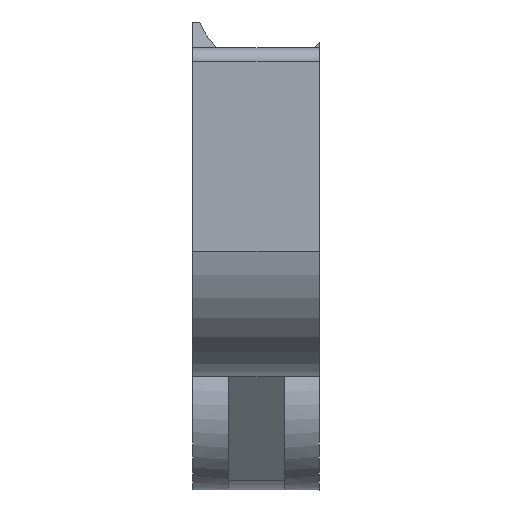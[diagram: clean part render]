
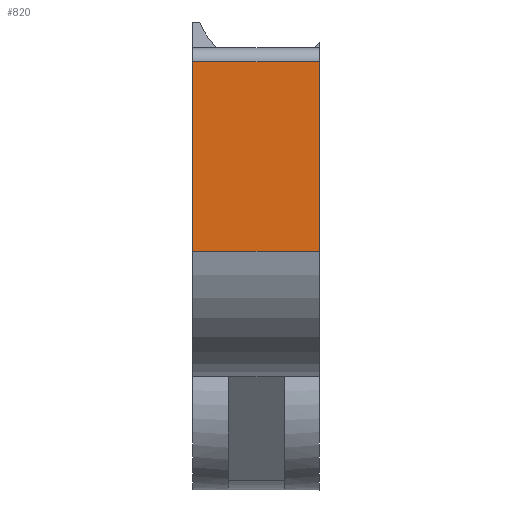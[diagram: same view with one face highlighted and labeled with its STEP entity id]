
A CAD part, left-side view. The second image highlights one B-rep face of the part: STEP entity #820.
In plain terms, the highlighted planar face has unit normal (-1, 0, 0).
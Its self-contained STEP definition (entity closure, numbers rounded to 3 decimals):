
#2 = DIRECTION ( 'NONE',  ( 0., -1., 0. ) ) ;
#34 = PLANE ( 'NONE',  #35 ) ;
#35 = AXIS2_PLACEMENT_3D ( 'NONE', #679, #856, #134 ) ;
#114 = EDGE_CURVE ( 'NONE', #207, #745, #587, .T. ) ;
#118 = DIRECTION ( 'NONE',  ( 0., 0., -1. ) ) ;
#122 = VECTOR ( 'NONE', #557, 1000. ) ;
#124 = ORIENTED_EDGE ( 'NONE', *, *, #149, .T. ) ;
#130 = VERTEX_POINT ( 'NONE', #916 ) ;
#133 = CARTESIAN_POINT ( 'NONE',  ( -142.325, 28.65, -19.64 ) ) ;
#134 = DIRECTION ( 'NONE',  ( 0., 0., -1. ) ) ;
#149 = EDGE_CURVE ( 'NONE', #207, #130, #364, .T. ) ;
#180 = VECTOR ( 'NONE', #118, 1000. ) ;
#207 = VERTEX_POINT ( 'NONE', #276 ) ;
#276 = CARTESIAN_POINT ( 'NONE',  ( -142.325, 28.65, -6.13 ) ) ;
#279 = FACE_OUTER_BOUND ( 'NONE', #1028, .T. ) ;
#345 = VERTEX_POINT ( 'NONE', #1119 ) ;
#350 = EDGE_CURVE ( 'NONE', #745, #345, #1077, .T. ) ;
#364 = LINE ( 'NONE', #632, #122 ) ;
#395 = EDGE_CURVE ( 'NONE', #345, #130, #640, .T. ) ;
#437 = CARTESIAN_POINT ( 'NONE',  ( -142.325, 19.6, -6.13 ) ) ;
#485 = CARTESIAN_POINT ( 'NONE',  ( -142.325, 19.6, -14.154 ) ) ;
#499 = DIRECTION ( 'NONE',  ( 0., 1., 0. ) ) ;
#530 = CARTESIAN_POINT ( 'NONE',  ( -142.325, 25.6, -6.13 ) ) ;
#545 = ORIENTED_EDGE ( 'NONE', *, *, #395, .F. ) ;
#557 = DIRECTION ( 'NONE',  ( 0., 0., -1. ) ) ;
#587 = LINE ( 'NONE', #530, #1161 ) ;
#632 = CARTESIAN_POINT ( 'NONE',  ( -142.325, 28.65, -16.707 ) ) ;
#640 = LINE ( 'NONE', #133, #1095 ) ;
#644 = ORIENTED_EDGE ( 'NONE', *, *, #114, .F. ) ;
#666 = ORIENTED_EDGE ( 'NONE', *, *, #350, .F. ) ;
#679 = CARTESIAN_POINT ( 'NONE',  ( -142.325, 23.6, -12.385 ) ) ;
#745 = VERTEX_POINT ( 'NONE', #437 ) ;
#820 = ADVANCED_FACE ( 'NONE', ( #279 ), #34, .F. ) ;
#856 = DIRECTION ( 'NONE',  ( 1., 0., 0. ) ) ;
#916 = CARTESIAN_POINT ( 'NONE',  ( -142.325, 28.65, -19.64 ) ) ;
#1028 = EDGE_LOOP ( 'NONE', ( #644, #124, #545, #666 ) ) ;
#1077 = LINE ( 'NONE', #485, #180 ) ;
#1095 = VECTOR ( 'NONE', #499, 1000. ) ;
#1119 = CARTESIAN_POINT ( 'NONE',  ( -142.325, 19.6, -19.64 ) ) ;
#1161 = VECTOR ( 'NONE', #2, 1000. ) ;
